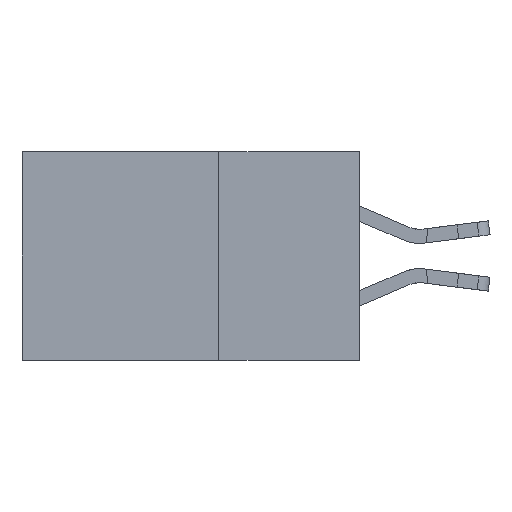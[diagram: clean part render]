
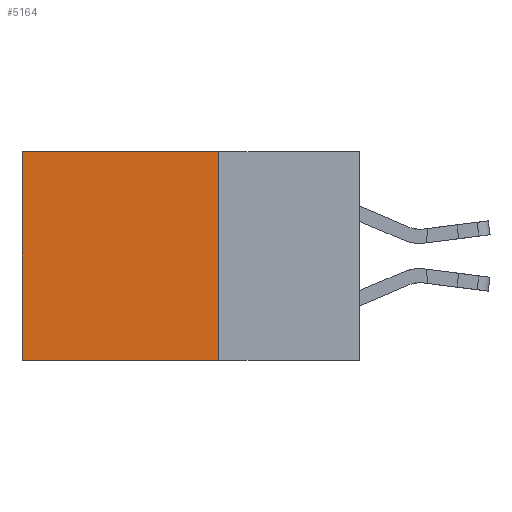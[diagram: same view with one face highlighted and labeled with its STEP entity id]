
A CAD part, left-side view. The second image highlights one B-rep face of the part: STEP entity #5164.
In plain terms, the highlighted planar face has unit normal (-1, 0, 0).
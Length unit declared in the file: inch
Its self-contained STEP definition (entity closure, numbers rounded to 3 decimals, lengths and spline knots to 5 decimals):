
#84 = DIRECTION ( 'NONE',  ( 0., 1., 0. ) ) ;
#380 = ORIENTED_EDGE ( 'NONE', *, *, #9703, .T. ) ;
#1290 = EDGE_CURVE ( 'NONE', #3672, #13937, #13417, .T. ) ;
#1418 = DIRECTION ( 'NONE',  ( 0., 1., 0. ) ) ;
#1677 = VECTOR ( 'NONE', #13157, 39.37008 ) ;
#2049 = ORIENTED_EDGE ( 'NONE', *, *, #20738, .F. ) ;
#2361 = ORIENTED_EDGE ( 'NONE', *, *, #4098, .F. ) ;
#2410 = CARTESIAN_POINT ( 'NONE',  ( 0.2875, 0.25, 0. ) ) ;
#2939 = CARTESIAN_POINT ( 'NONE',  ( 0.2875, 0.25, 0. ) ) ;
#3070 = CARTESIAN_POINT ( 'NONE',  ( 0.2875, 0.6, 0. ) ) ;
#3665 = CARTESIAN_POINT ( 'NONE',  ( 0.2875, 0.25, 0. ) ) ;
#3672 = VERTEX_POINT ( 'NONE', #2410 ) ;
#4098 = EDGE_CURVE ( 'NONE', #3672, #16357, #12250, .T. ) ;
#4514 = EDGE_LOOP ( 'NONE', ( #380, #2049, #2361, #5637 ) ) ;
#4922 = CARTESIAN_POINT ( 'NONE',  ( 0.2875, 0.6, 0. ) ) ;
#5164 = ADVANCED_FACE ( 'NONE', ( #17763 ), #5961, .F. ) ;
#5407 = CARTESIAN_POINT ( 'NONE',  ( 0.2875, 0.25, -0.37 ) ) ;
#5637 = ORIENTED_EDGE ( 'NONE', *, *, #1290, .T. ) ;
#5961 = PLANE ( 'NONE',  #17746 ) ;
#6065 = DIRECTION ( 'NONE',  ( 1., 0., 0. ) ) ;
#9703 = EDGE_CURVE ( 'NONE', #13937, #14537, #19729, .T. ) ;
#10406 = DIRECTION ( 'NONE',  ( 0., 0., -1. ) ) ;
#11734 = CARTESIAN_POINT ( 'NONE',  ( 0.2875, 0.6, -0.37 ) ) ;
#12250 = LINE ( 'NONE', #3665, #12920 ) ;
#12900 = LINE ( 'NONE', #16211, #17226 ) ;
#12920 = VECTOR ( 'NONE', #10406, 39.37008 ) ;
#13157 = DIRECTION ( 'NONE',  ( 0., 0., -1. ) ) ;
#13417 = LINE ( 'NONE', #18254, #13855 ) ;
#13855 = VECTOR ( 'NONE', #84, 39.37008 ) ;
#13937 = VERTEX_POINT ( 'NONE', #3070 ) ;
#14537 = VERTEX_POINT ( 'NONE', #11734 ) ;
#16124 = DIRECTION ( 'NONE',  ( 0., 0., -1. ) ) ;
#16211 = CARTESIAN_POINT ( 'NONE',  ( 0.2875, 0.25, -0.37 ) ) ;
#16357 = VERTEX_POINT ( 'NONE', #5407 ) ;
#17226 = VECTOR ( 'NONE', #1418, 39.37008 ) ;
#17746 = AXIS2_PLACEMENT_3D ( 'NONE', #2939, #6065, #16124 ) ;
#17763 = FACE_OUTER_BOUND ( 'NONE', #4514, .T. ) ;
#18254 = CARTESIAN_POINT ( 'NONE',  ( 0.2875, 0.25, 0. ) ) ;
#19729 = LINE ( 'NONE', #4922, #1677 ) ;
#20738 = EDGE_CURVE ( 'NONE', #16357, #14537, #12900, .T. ) ;
